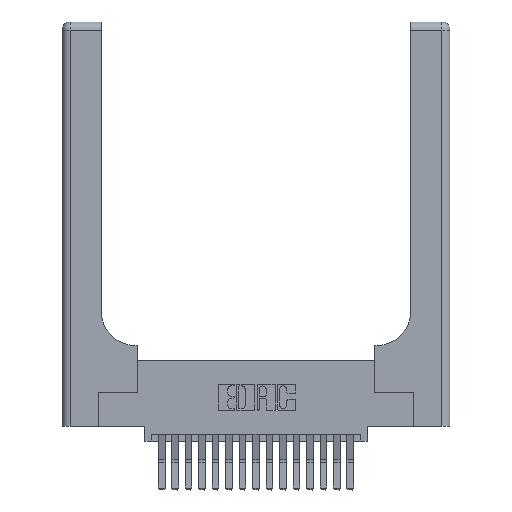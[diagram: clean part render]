
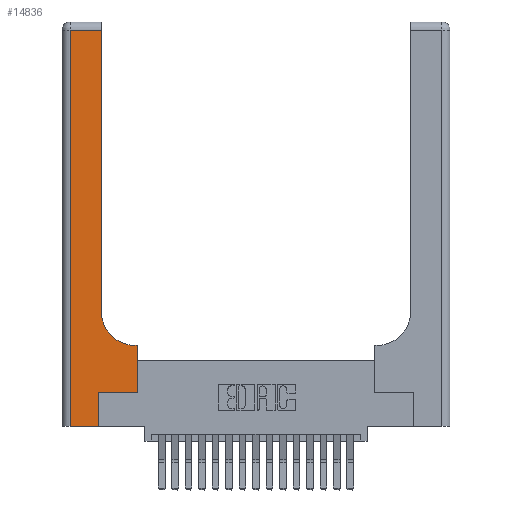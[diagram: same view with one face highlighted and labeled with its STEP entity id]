
A CAD part, top view. The second image highlights one B-rep face of the part: STEP entity #14836.
In plain terms, the highlighted planar face has unit normal (0, 0, 1).
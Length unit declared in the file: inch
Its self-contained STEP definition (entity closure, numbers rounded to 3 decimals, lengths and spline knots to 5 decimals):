
#250 = CARTESIAN_POINT ( 'NONE',  ( 0.2915, 0.85, 0.37 ) ) ;
#834 = EDGE_CURVE ( 'NONE', #12483, #18314, #8346, .T. ) ;
#1092 = LINE ( 'NONE', #16902, #9179 ) ;
#1155 = CARTESIAN_POINT ( 'NONE',  ( 0.06, 3., 0.37 ) ) ;
#1191 = VERTEX_POINT ( 'NONE', #3567 ) ;
#1354 = ORIENTED_EDGE ( 'NONE', *, *, #3300, .T. ) ;
#1551 = DIRECTION ( 'NONE',  ( 0., 0., -1. ) ) ;
#1885 = VECTOR ( 'NONE', #5671, 39.37008 ) ;
#2041 = VERTEX_POINT ( 'NONE', #10018 ) ;
#3300 = EDGE_CURVE ( 'NONE', #14206, #1191, #11552, .T. ) ;
#3567 = CARTESIAN_POINT ( 'NONE',  ( 0.06, 2.94, 0.37 ) ) ;
#4054 = CARTESIAN_POINT ( 'NONE',  ( 0.2915, 3., 0.37 ) ) ;
#4127 = DIRECTION ( 'NONE',  ( 0., 1., 0. ) ) ;
#4217 = LINE ( 'NONE', #19264, #16553 ) ;
#4517 = VERTEX_POINT ( 'NONE', #19537 ) ;
#5648 = AXIS2_PLACEMENT_3D ( 'NONE', #8964, #20186, #10609 ) ;
#5671 = DIRECTION ( 'NONE',  ( 0., 1., 0. ) ) ;
#6435 = ORIENTED_EDGE ( 'NONE', *, *, #15961, .T. ) ;
#6585 = CARTESIAN_POINT ( 'NONE',  ( 0.269, 0., 0.37 ) ) ;
#6944 = ORIENTED_EDGE ( 'NONE', *, *, #15280, .T. ) ;
#7246 = VECTOR ( 'NONE', #8753, 39.37008 ) ;
#7251 = VERTEX_POINT ( 'NONE', #15045 ) ;
#8014 = DIRECTION ( 'NONE',  ( -1., 0., 0. ) ) ;
#8238 = DIRECTION ( 'NONE',  ( 1., 0., 0. ) ) ;
#8346 = LINE ( 'NONE', #8416, #11657 ) ;
#8416 = CARTESIAN_POINT ( 'NONE',  ( 0., 0., 0.37 ) ) ;
#8695 = FACE_OUTER_BOUND ( 'NONE', #17901, .T. ) ;
#8753 = DIRECTION ( 'NONE',  ( -1., 0., 0. ) ) ;
#8806 = EDGE_CURVE ( 'NONE', #4517, #7251, #4217, .T. ) ;
#8940 = ORIENTED_EDGE ( 'NONE', *, *, #11940, .T. ) ;
#8964 = CARTESIAN_POINT ( 'NONE',  ( 0.5415, 0.85, 0.37 ) ) ;
#9179 = VECTOR ( 'NONE', #18519, 39.37008 ) ;
#9465 = LINE ( 'NONE', #15296, #1885 ) ;
#9589 = CIRCLE ( 'NONE', #5648, 0.25 ) ;
#9802 = EDGE_CURVE ( 'NONE', #1191, #12483, #20739, .T. ) ;
#10018 = CARTESIAN_POINT ( 'NONE',  ( 0.5585, 0.25, 0.37 ) ) ;
#10183 = EDGE_CURVE ( 'NONE', #18314, #14574, #9465, .T. ) ;
#10325 = AXIS2_PLACEMENT_3D ( 'NONE', #15972, #1551, #12836 ) ;
#10609 = DIRECTION ( 'NONE',  ( 1., 0., 0. ) ) ;
#10617 = CARTESIAN_POINT ( 'NONE',  ( 0.269, 0.25, 0.37 ) ) ;
#10635 = DIRECTION ( 'NONE',  ( 1., 0., 0. ) ) ;
#10852 = DIRECTION ( 'NONE',  ( 0., -1., 0. ) ) ;
#11243 = PLANE ( 'NONE',  #10325 ) ;
#11249 = ORIENTED_EDGE ( 'NONE', *, *, #8806, .T. ) ;
#11552 = LINE ( 'NONE', #18393, #7246 ) ;
#11583 = LINE ( 'NONE', #4054, #14304 ) ;
#11657 = VECTOR ( 'NONE', #8238, 39.37008 ) ;
#11940 = EDGE_CURVE ( 'NONE', #15693, #14206, #11583, .T. ) ;
#12269 = VECTOR ( 'NONE', #10852, 39.37008 ) ;
#12449 = CARTESIAN_POINT ( 'NONE',  ( 0.2915, 2.94, 0.37 ) ) ;
#12483 = VERTEX_POINT ( 'NONE', #19440 ) ;
#12836 = DIRECTION ( 'NONE',  ( -1., 0., 0. ) ) ;
#14177 = VECTOR ( 'NONE', #10635, 39.37008 ) ;
#14206 = VERTEX_POINT ( 'NONE', #12449 ) ;
#14304 = VECTOR ( 'NONE', #4127, 39.37008 ) ;
#14574 = VERTEX_POINT ( 'NONE', #10617 ) ;
#14836 = ADVANCED_FACE ( 'NONE', ( #8695 ), #11243, .F. ) ;
#15045 = CARTESIAN_POINT ( 'NONE',  ( 0.5415, 0.6, 0.37 ) ) ;
#15280 = EDGE_CURVE ( 'NONE', #2041, #4517, #1092, .T. ) ;
#15296 = CARTESIAN_POINT ( 'NONE',  ( 0.269, 0., 0.37 ) ) ;
#15693 = VERTEX_POINT ( 'NONE', #250 ) ;
#15961 = EDGE_CURVE ( 'NONE', #14574, #2041, #18954, .T. ) ;
#15972 = CARTESIAN_POINT ( 'NONE',  ( 0., 3., 0.37 ) ) ;
#16553 = VECTOR ( 'NONE', #8014, 39.37008 ) ;
#16902 = CARTESIAN_POINT ( 'NONE',  ( 0.5585, 0.25, 0.37 ) ) ;
#17901 = EDGE_LOOP ( 'NONE', ( #8940, #1354, #19235, #19489, #20483, #6435, #6944, #11249, #19757 ) ) ;
#18314 = VERTEX_POINT ( 'NONE', #6585 ) ;
#18393 = CARTESIAN_POINT ( 'NONE',  ( 0., 2.94, 0.37 ) ) ;
#18519 = DIRECTION ( 'NONE',  ( 0., 1., 0. ) ) ;
#18954 = LINE ( 'NONE', #20217, #14177 ) ;
#19235 = ORIENTED_EDGE ( 'NONE', *, *, #9802, .T. ) ;
#19264 = CARTESIAN_POINT ( 'NONE',  ( 0.2915, 0.6, 0.37 ) ) ;
#19440 = CARTESIAN_POINT ( 'NONE',  ( 0.06, 0., 0.37 ) ) ;
#19489 = ORIENTED_EDGE ( 'NONE', *, *, #834, .T. ) ;
#19537 = CARTESIAN_POINT ( 'NONE',  ( 0.5585, 0.6, 0.37 ) ) ;
#19757 = ORIENTED_EDGE ( 'NONE', *, *, #20530, .T. ) ;
#20186 = DIRECTION ( 'NONE',  ( 0., 0., -1. ) ) ;
#20217 = CARTESIAN_POINT ( 'NONE',  ( 0.269, 0.25, 0.37 ) ) ;
#20483 = ORIENTED_EDGE ( 'NONE', *, *, #10183, .T. ) ;
#20530 = EDGE_CURVE ( 'NONE', #7251, #15693, #9589, .T. ) ;
#20739 = LINE ( 'NONE', #1155, #12269 ) ;
